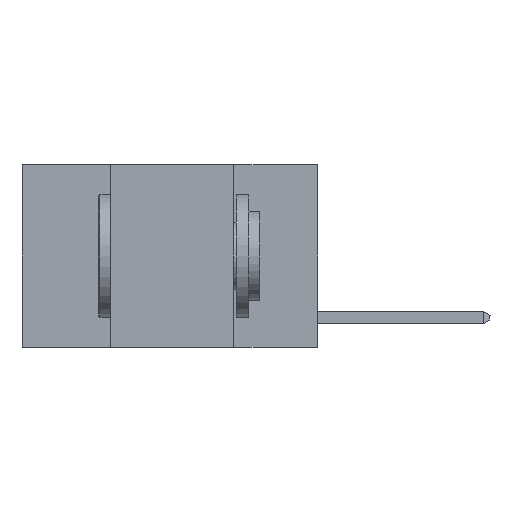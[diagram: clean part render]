
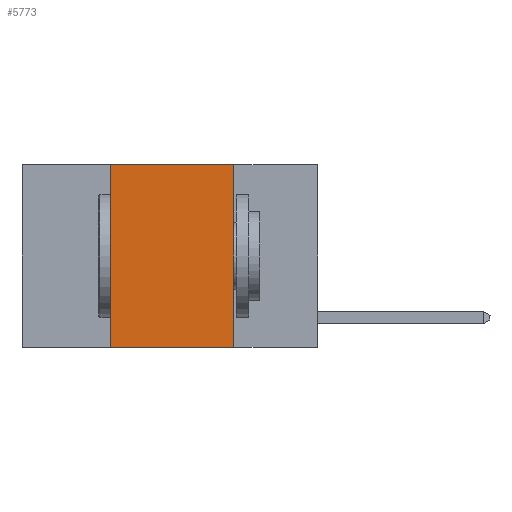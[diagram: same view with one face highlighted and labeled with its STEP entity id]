
A CAD part, left-side view. The second image highlights one B-rep face of the part: STEP entity #5773.
In plain terms, the highlighted planar face has unit normal (-1, 0, 0).
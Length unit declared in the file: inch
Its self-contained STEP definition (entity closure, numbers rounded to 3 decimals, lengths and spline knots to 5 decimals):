
#319 = EDGE_CURVE ( 'NONE', #5446, #11904, #8425, .T. ) ;
#475 = CARTESIAN_POINT ( 'NONE',  ( 0., 0.42, 0. ) ) ;
#733 = LINE ( 'NONE', #7437, #3652 ) ;
#2025 = FACE_OUTER_BOUND ( 'NONE', #4131, .T. ) ;
#2451 = DIRECTION ( 'NONE',  ( 0., -1., 0. ) ) ;
#2811 = VECTOR ( 'NONE', #10336, 39.37008 ) ;
#3013 = AXIS2_PLACEMENT_3D ( 'NONE', #10978, #6055, #6116 ) ;
#3290 = ORIENTED_EDGE ( 'NONE', *, *, #11965, .F. ) ;
#3652 = VECTOR ( 'NONE', #2451, 39.37008 ) ;
#4131 = EDGE_LOOP ( 'NONE', ( #7995, #7720, #3290, #10520 ) ) ;
#4552 = LINE ( 'NONE', #11286, #2811 ) ;
#5445 = DIRECTION ( 'NONE',  ( 0., -1., 0. ) ) ;
#5446 = VERTEX_POINT ( 'NONE', #8109 ) ;
#5773 = ADVANCED_FACE ( 'NONE', ( #2025 ), #11873, .F. ) ;
#5852 = EDGE_CURVE ( 'NONE', #7627, #6542, #733, .T. ) ;
#5925 = EDGE_CURVE ( 'NONE', #6542, #11904, #4552, .T. ) ;
#6055 = DIRECTION ( 'NONE',  ( 1., 0., 0. ) ) ;
#6116 = DIRECTION ( 'NONE',  ( 0., 0., -1. ) ) ;
#6542 = VERTEX_POINT ( 'NONE', #7671 ) ;
#7437 = CARTESIAN_POINT ( 'NONE',  ( 0., 0.6, 0. ) ) ;
#7452 = CARTESIAN_POINT ( 'NONE',  ( 0., 0.6, -0.37 ) ) ;
#7627 = VERTEX_POINT ( 'NONE', #475 ) ;
#7671 = CARTESIAN_POINT ( 'NONE',  ( 0., 0.17, 0. ) ) ;
#7720 = ORIENTED_EDGE ( 'NONE', *, *, #5852, .F. ) ;
#7995 = ORIENTED_EDGE ( 'NONE', *, *, #5925, .F. ) ;
#8108 = CARTESIAN_POINT ( 'NONE',  ( 0., 0.17, -0.37 ) ) ;
#8109 = CARTESIAN_POINT ( 'NONE',  ( 0., 0.42, -0.37 ) ) ;
#8425 = LINE ( 'NONE', #7452, #12175 ) ;
#9539 = DIRECTION ( 'NONE',  ( 0., 0., 1. ) ) ;
#10336 = DIRECTION ( 'NONE',  ( 0., 0., -1. ) ) ;
#10520 = ORIENTED_EDGE ( 'NONE', *, *, #319, .T. ) ;
#10795 = VECTOR ( 'NONE', #9539, 39.37008 ) ;
#10978 = CARTESIAN_POINT ( 'NONE',  ( 0., 0.6, 0. ) ) ;
#11286 = CARTESIAN_POINT ( 'NONE',  ( 0., 0.17, 0. ) ) ;
#11514 = CARTESIAN_POINT ( 'NONE',  ( 0., 0.42, 0. ) ) ;
#11873 = PLANE ( 'NONE',  #3013 ) ;
#11904 = VERTEX_POINT ( 'NONE', #8108 ) ;
#11965 = EDGE_CURVE ( 'NONE', #5446, #7627, #12453, .T. ) ;
#12175 = VECTOR ( 'NONE', #5445, 39.37008 ) ;
#12453 = LINE ( 'NONE', #11514, #10795 ) ;
